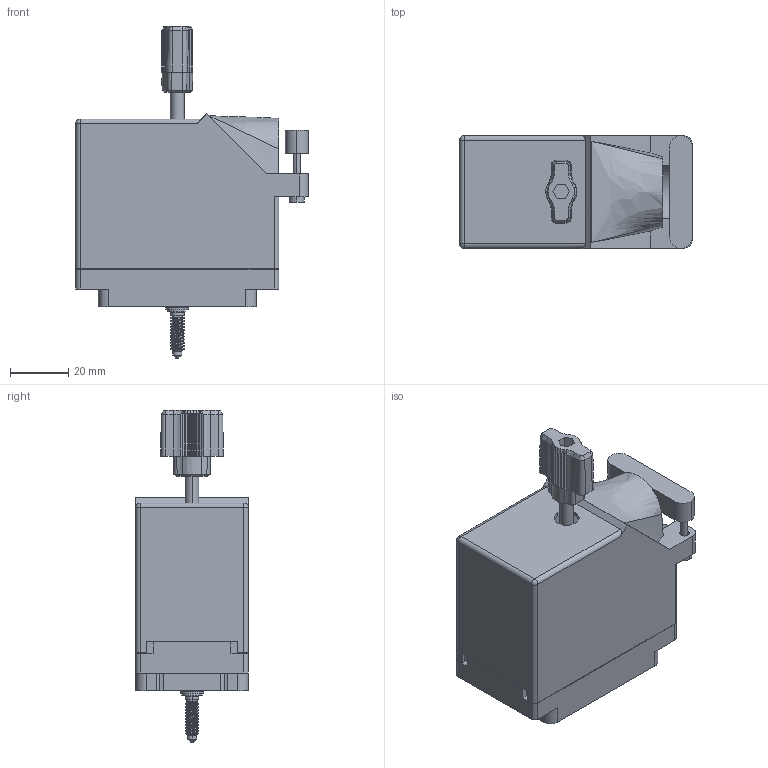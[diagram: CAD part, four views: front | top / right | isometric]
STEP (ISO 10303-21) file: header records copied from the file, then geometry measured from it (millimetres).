
FILE_DESCRIPTION (( 'STEP AP203' ), '1' );
FILE_NAME ('516-120-000-325.STEP', '2020-03-11T01:36:10', ( '' ), ( '' ), 'SwSTEP 2.0', 'SolidWorks 2016', '' );
FILE_SCHEMA (( 'CONFIG_CONTROL_DESIGN' ));
Length unit declared in the file: inch
Products named in the file (10): 516 Plug Insulator_120; 516-250-091-111; 516-120-000-325; Actuating Screw Assy 090-120; 516-254-091-109; Grub Screw; 516-230-001_Plastic - 120 Side Entry; 516-253-190-107; 516-253-095-100; 516-251-095-100
Assembly tree (10 placements, depth 3):
  516-120-000-325
    516 Plug Insulator_120
    516-230-001_Plastic - 120 Side Entry
    Actuating Screw Assy 090-120
      516-251-095-100
      516-254-091-109
      516-253-095-100  x2
      516-253-190-107
      516-250-091-111
      Grub Screw
Bounding box: 80.14 x 38.86 x 114.34 mm (x, y, z)
Volume: 47105.3 mm3; surface area: 58865.1 mm2
Topology: 9 solids, 9 shells, 2752 faces, 8039 edges, 5328 vertices
Faces by surface type: plane 1948, cylinder 720, cone 62, bspline 20, sphere 2
Entity records: 99262 total; most frequent: CARTESIAN_POINT 23496, ORIENTED_EDGE 16050, DIRECTION 15226, EDGE_CURVE 8025, VECTOR 5902, LINE 5902, VERTEX_POINT 5320, AXIS2_PLACEMENT_3D 4662
